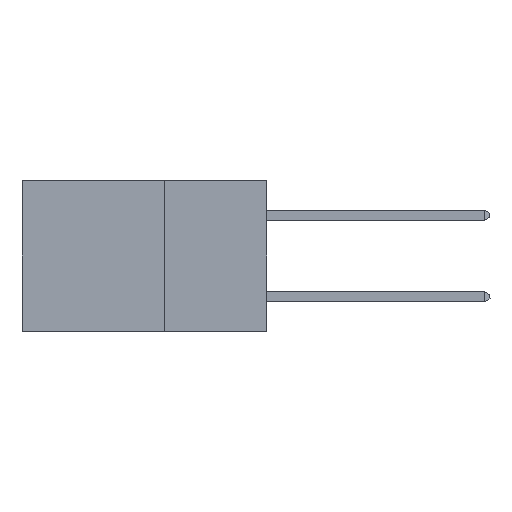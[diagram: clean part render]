
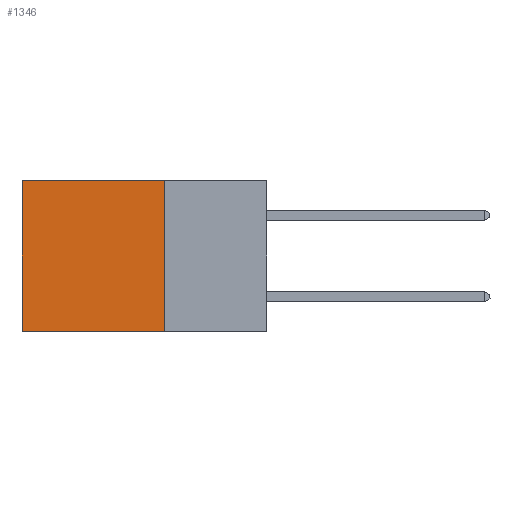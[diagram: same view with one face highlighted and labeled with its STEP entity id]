
A CAD part, left-side view. The second image highlights one B-rep face of the part: STEP entity #1346.
In plain terms, the highlighted planar face has unit normal (-1, 0, 0).
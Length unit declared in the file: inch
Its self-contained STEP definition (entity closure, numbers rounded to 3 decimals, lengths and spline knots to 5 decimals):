
#190 = ORIENTED_EDGE ( 'NONE', *, *, #15223, .T. ) ;
#863 = ORIENTED_EDGE ( 'NONE', *, *, #2752, .F. ) ;
#1346 = ADVANCED_FACE ( 'NONE', ( #15509 ), #9337, .F. ) ;
#1769 = DIRECTION ( 'NONE',  ( 0., 1., 0. ) ) ;
#1813 = VECTOR ( 'NONE', #1769, 39.37008 ) ;
#2716 = CARTESIAN_POINT ( 'NONE',  ( 0.2875, 0.6, 0. ) ) ;
#2752 = EDGE_CURVE ( 'NONE', #14670, #12852, #17923, .T. ) ;
#4755 = CARTESIAN_POINT ( 'NONE',  ( 0.2875, 0.6, -0.37 ) ) ;
#5475 = DIRECTION ( 'NONE',  ( 1., 0., 0. ) ) ;
#6077 = CARTESIAN_POINT ( 'NONE',  ( 0.2875, 0.25, -0.37 ) ) ;
#6345 = CARTESIAN_POINT ( 'NONE',  ( 0.2875, 0.25, -0.37 ) ) ;
#6436 = AXIS2_PLACEMENT_3D ( 'NONE', #16960, #5475, #22709 ) ;
#6551 = CARTESIAN_POINT ( 'NONE',  ( 0.2875, 0.25, 0. ) ) ;
#6885 = EDGE_CURVE ( 'NONE', #15823, #12852, #14491, .T. ) ;
#9337 = PLANE ( 'NONE',  #6436 ) ;
#9421 = CARTESIAN_POINT ( 'NONE',  ( 0.2875, 0.25, 0. ) ) ;
#10103 = VERTEX_POINT ( 'NONE', #6551 ) ;
#10292 = ORIENTED_EDGE ( 'NONE', *, *, #11226, .F. ) ;
#10772 = VECTOR ( 'NONE', #21355, 39.37008 ) ;
#11226 = EDGE_CURVE ( 'NONE', #10103, #14670, #23639, .T. ) ;
#12852 = VERTEX_POINT ( 'NONE', #4755 ) ;
#13447 = LINE ( 'NONE', #9421, #1813 ) ;
#13891 = VECTOR ( 'NONE', #21942, 39.37008 ) ;
#14491 = LINE ( 'NONE', #2716, #13891 ) ;
#14670 = VERTEX_POINT ( 'NONE', #6077 ) ;
#15223 = EDGE_CURVE ( 'NONE', #10103, #15823, #13447, .T. ) ;
#15306 = ORIENTED_EDGE ( 'NONE', *, *, #6885, .T. ) ;
#15509 = FACE_OUTER_BOUND ( 'NONE', #18407, .T. ) ;
#15823 = VERTEX_POINT ( 'NONE', #22413 ) ;
#16215 = DIRECTION ( 'NONE',  ( 0., 0., -1. ) ) ;
#16960 = CARTESIAN_POINT ( 'NONE',  ( 0.2875, 0.25, 0. ) ) ;
#17750 = CARTESIAN_POINT ( 'NONE',  ( 0.2875, 0.25, 0. ) ) ;
#17923 = LINE ( 'NONE', #6345, #10772 ) ;
#18407 = EDGE_LOOP ( 'NONE', ( #15306, #863, #10292, #190 ) ) ;
#21355 = DIRECTION ( 'NONE',  ( 0., 1., 0. ) ) ;
#21942 = DIRECTION ( 'NONE',  ( 0., 0., -1. ) ) ;
#22413 = CARTESIAN_POINT ( 'NONE',  ( 0.2875, 0.6, 0. ) ) ;
#22709 = DIRECTION ( 'NONE',  ( 0., 0., -1. ) ) ;
#23639 = LINE ( 'NONE', #17750, #24509 ) ;
#24509 = VECTOR ( 'NONE', #16215, 39.37008 ) ;
